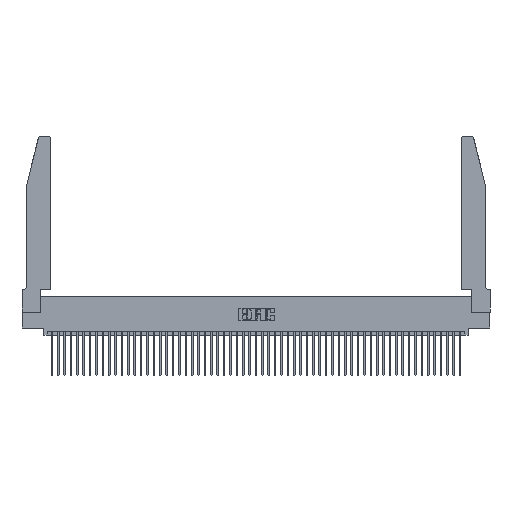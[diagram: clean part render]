
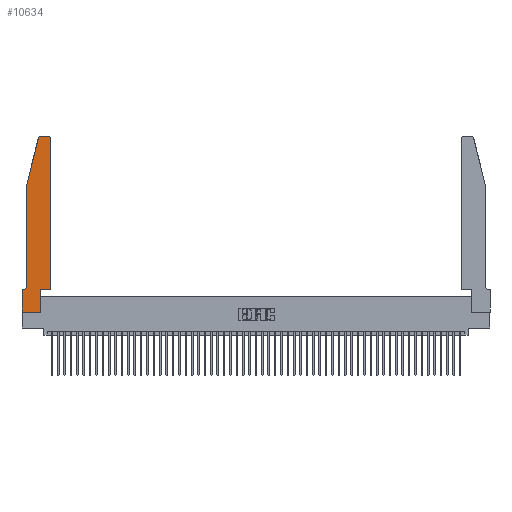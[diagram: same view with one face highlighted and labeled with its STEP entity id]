
A CAD part, top view. The second image highlights one B-rep face of the part: STEP entity #10634.
In plain terms, the highlighted planar face has unit normal (0, 0, 1).
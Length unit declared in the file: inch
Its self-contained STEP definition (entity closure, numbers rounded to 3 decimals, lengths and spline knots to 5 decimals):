
#159 = ORIENTED_EDGE ( 'NONE', *, *, #37753, .T. ) ;
#338 = LINE ( 'NONE', #2119, #4247 ) ;
#1248 = LINE ( 'NONE', #48090, #3848 ) ;
#1763 = ORIENTED_EDGE ( 'NONE', *, *, #9691, .T. ) ;
#2119 = CARTESIAN_POINT ( 'NONE',  ( 0.2605, 2.75, 0.37 ) ) ;
#3101 = EDGE_CURVE ( 'NONE', #46702, #41114, #39444, .T. ) ;
#3848 = VECTOR ( 'NONE', #43836, 39.37008 ) ;
#3914 = DIRECTION ( 'NONE',  ( 0., 0., 1. ) ) ;
#4247 = VECTOR ( 'NONE', #34428, 39.37008 ) ;
#4481 = DIRECTION ( 'NONE',  ( 1., 0., 0. ) ) ;
#4628 = DIRECTION ( 'NONE',  ( 0., -1., 0. ) ) ;
#5580 = DIRECTION ( 'NONE',  ( 1., 0., 0. ) ) ;
#6011 = VECTOR ( 'NONE', #41809, 39.37008 ) ;
#6343 = CIRCLE ( 'NONE', #11067, 0.07 ) ;
#6667 = LINE ( 'NONE', #9743, #6011 ) ;
#6818 = VERTEX_POINT ( 'NONE', #19630 ) ;
#7025 = CARTESIAN_POINT ( 'NONE',  ( 0., 0., 0.37 ) ) ;
#7082 = CARTESIAN_POINT ( 'NONE',  ( 0., 0., 0.37 ) ) ;
#7375 = VERTEX_POINT ( 'NONE', #7082 ) ;
#7433 = CARTESIAN_POINT ( 'NONE',  ( 0.284, 2.75, 0.37 ) ) ;
#7958 = CARTESIAN_POINT ( 'NONE',  ( 0.4505, 0.35, 0.37 ) ) ;
#8672 = EDGE_CURVE ( 'NONE', #32315, #21783, #12271, .T. ) ;
#8830 = EDGE_LOOP ( 'NONE', ( #8851, #51085, #42395, #25721, #19863, #34358, #47875, #1763, #19983, #23265, #49844, #159 ) ) ;
#8851 = ORIENTED_EDGE ( 'NONE', *, *, #40516, .T. ) ;
#9463 = DIRECTION ( 'NONE',  ( 0., 0., 1. ) ) ;
#9691 = EDGE_CURVE ( 'NONE', #7375, #46702, #21763, .T. ) ;
#9743 = CARTESIAN_POINT ( 'NONE',  ( 0.4505, 0.35, 0.37 ) ) ;
#10634 = ADVANCED_FACE ( 'NONE', ( #19704 ), #17311, .T. ) ;
#10934 = DIRECTION ( 'NONE',  ( 1., 0., 0. ) ) ;
#11067 = AXIS2_PLACEMENT_3D ( 'NONE', #31006, #51084, #39675 ) ;
#12263 = DIRECTION ( 'NONE',  ( 0., -1., 0. ) ) ;
#12271 = CIRCLE ( 'NONE', #41521, 0.03 ) ;
#12970 = VERTEX_POINT ( 'NONE', #7958 ) ;
#13718 = CARTESIAN_POINT ( 'NONE',  ( 0.0755, 0.42, 0.37 ) ) ;
#15506 = VECTOR ( 'NONE', #47342, 39.37008 ) ;
#16797 = LINE ( 'NONE', #38815, #15506 ) ;
#17151 = EDGE_CURVE ( 'NONE', #21783, #26209, #1248, .T. ) ;
#17311 = PLANE ( 'NONE',  #39176 ) ;
#18189 = VECTOR ( 'NONE', #12263, 39.37008 ) ;
#19260 = VERTEX_POINT ( 'NONE', #50025 ) ;
#19397 = CARTESIAN_POINT ( 'NONE',  ( 0.2865, 0., 0.37 ) ) ;
#19630 = CARTESIAN_POINT ( 'NONE',  ( 0.4505, 2.72, 0.37 ) ) ;
#19704 = FACE_OUTER_BOUND ( 'NONE', #8830, .T. ) ;
#19863 = ORIENTED_EDGE ( 'NONE', *, *, #39127, .T. ) ;
#19983 = ORIENTED_EDGE ( 'NONE', *, *, #3101, .T. ) ;
#20150 = DIRECTION ( 'NONE',  ( 1., 0., 0. ) ) ;
#20206 = CARTESIAN_POINT ( 'NONE',  ( 0.2865, 0.35, 0.37 ) ) ;
#20481 = VECTOR ( 'NONE', #10934, 39.37008 ) ;
#20887 = CARTESIAN_POINT ( 'NONE',  ( 0.284, 2.72, 0.37 ) ) ;
#21048 = EDGE_CURVE ( 'NONE', #26209, #38960, #22040, .T. ) ;
#21333 = EDGE_CURVE ( 'NONE', #41114, #12970, #6667, .T. ) ;
#21763 = LINE ( 'NONE', #7025, #20481 ) ;
#21783 = VERTEX_POINT ( 'NONE', #49592 ) ;
#22040 = LINE ( 'NONE', #37489, #18189 ) ;
#23265 = ORIENTED_EDGE ( 'NONE', *, *, #21333, .T. ) ;
#24056 = EDGE_CURVE ( 'NONE', #34661, #7375, #41423, .T. ) ;
#25519 = CIRCLE ( 'NONE', #45185, 0.03 ) ;
#25721 = ORIENTED_EDGE ( 'NONE', *, *, #21048, .T. ) ;
#26163 = VECTOR ( 'NONE', #4628, 39.37008 ) ;
#26209 = VERTEX_POINT ( 'NONE', #26523 ) ;
#26268 = VECTOR ( 'NONE', #29964, 39.37008 ) ;
#26523 = CARTESIAN_POINT ( 'NONE',  ( 0.0755, 2., 0.37 ) ) ;
#29964 = DIRECTION ( 'NONE',  ( -1., 0., 0. ) ) ;
#30228 = EDGE_CURVE ( 'NONE', #12970, #6818, #16797, .T. ) ;
#30491 = VERTEX_POINT ( 'NONE', #32743 ) ;
#31006 = CARTESIAN_POINT ( 'NONE',  ( 0.0055, 0.42, 0.37 ) ) ;
#32315 = VERTEX_POINT ( 'NONE', #7433 ) ;
#32743 = CARTESIAN_POINT ( 'NONE',  ( 0.0055, 0.35, 0.37 ) ) ;
#34358 = ORIENTED_EDGE ( 'NONE', *, *, #42379, .T. ) ;
#34428 = DIRECTION ( 'NONE',  ( -1., 0., 0. ) ) ;
#34661 = VERTEX_POINT ( 'NONE', #41287 ) ;
#36529 = CARTESIAN_POINT ( 'NONE',  ( 0., 0.35, 0.37 ) ) ;
#36875 = CARTESIAN_POINT ( 'NONE',  ( 0., 0., 0.37 ) ) ;
#37489 = CARTESIAN_POINT ( 'NONE',  ( 0.0755, 2., 0.37 ) ) ;
#37753 = EDGE_CURVE ( 'NONE', #6818, #19260, #25519, .T. ) ;
#38099 = CARTESIAN_POINT ( 'NONE',  ( 0.2865, 0.35, 0.37 ) ) ;
#38815 = CARTESIAN_POINT ( 'NONE',  ( 0.4505, 0.35, 0.37 ) ) ;
#38960 = VERTEX_POINT ( 'NONE', #13718 ) ;
#39127 = EDGE_CURVE ( 'NONE', #38960, #30491, #6343, .T. ) ;
#39176 = AXIS2_PLACEMENT_3D ( 'NONE', #36529, #3914, #20150 ) ;
#39444 = LINE ( 'NONE', #20206, #41405 ) ;
#39675 = DIRECTION ( 'NONE',  ( -1., 0., 0. ) ) ;
#40516 = EDGE_CURVE ( 'NONE', #19260, #32315, #338, .T. ) ;
#41114 = VERTEX_POINT ( 'NONE', #38099 ) ;
#41287 = CARTESIAN_POINT ( 'NONE',  ( 0., 0.35, 0.37 ) ) ;
#41405 = VECTOR ( 'NONE', #52592, 39.37008 ) ;
#41423 = LINE ( 'NONE', #36875, #26163 ) ;
#41521 = AXIS2_PLACEMENT_3D ( 'NONE', #20887, #49345, #4481 ) ;
#41809 = DIRECTION ( 'NONE',  ( 1., 0., 0. ) ) ;
#41855 = CARTESIAN_POINT ( 'NONE',  ( 0.0755, 0.35, 0.37 ) ) ;
#42213 = CARTESIAN_POINT ( 'NONE',  ( 0.4205, 2.72, 0.37 ) ) ;
#42379 = EDGE_CURVE ( 'NONE', #30491, #34661, #51737, .T. ) ;
#42395 = ORIENTED_EDGE ( 'NONE', *, *, #17151, .T. ) ;
#43836 = DIRECTION ( 'NONE',  ( -0.239, -0.971, 0. ) ) ;
#45185 = AXIS2_PLACEMENT_3D ( 'NONE', #42213, #9463, #5580 ) ;
#46702 = VERTEX_POINT ( 'NONE', #19397 ) ;
#47342 = DIRECTION ( 'NONE',  ( 0., 1., 0. ) ) ;
#47875 = ORIENTED_EDGE ( 'NONE', *, *, #24056, .T. ) ;
#48090 = CARTESIAN_POINT ( 'NONE',  ( 0.0755, 2., 0.37 ) ) ;
#49345 = DIRECTION ( 'NONE',  ( 0., 0., 1. ) ) ;
#49592 = CARTESIAN_POINT ( 'NONE',  ( 0.25487, 2.72718, 0.37 ) ) ;
#49844 = ORIENTED_EDGE ( 'NONE', *, *, #30228, .T. ) ;
#50025 = CARTESIAN_POINT ( 'NONE',  ( 0.4205, 2.75, 0.37 ) ) ;
#51084 = DIRECTION ( 'NONE',  ( 0., 0., -1. ) ) ;
#51085 = ORIENTED_EDGE ( 'NONE', *, *, #8672, .T. ) ;
#51737 = LINE ( 'NONE', #41855, #26268 ) ;
#52592 = DIRECTION ( 'NONE',  ( 0., 1., 0. ) ) ;
